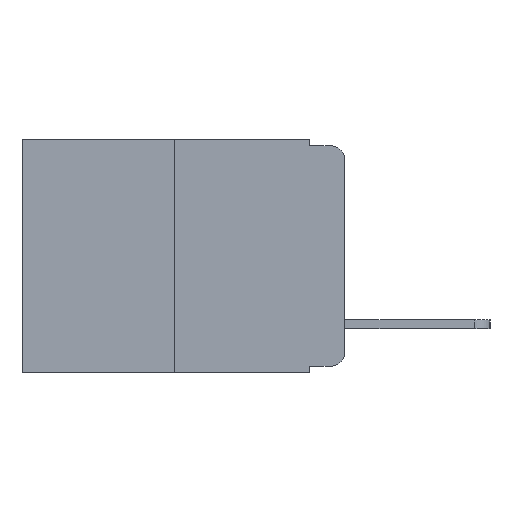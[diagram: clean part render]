
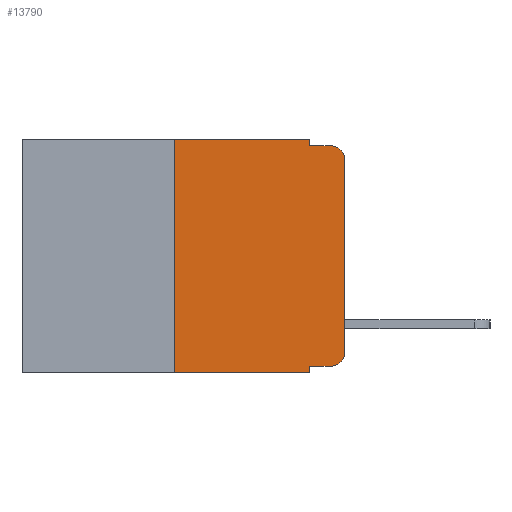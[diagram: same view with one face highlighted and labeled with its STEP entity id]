
A CAD part, left-side view. The second image highlights one B-rep face of the part: STEP entity #13790.
In plain terms, the highlighted planar face has unit normal (-1, 0, 0).
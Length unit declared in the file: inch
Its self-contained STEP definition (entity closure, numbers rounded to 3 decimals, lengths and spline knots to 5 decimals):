
#173 = CIRCLE ( 'NONE', #12057, 0.02 ) ;
#282 = CARTESIAN_POINT ( 'NONE',  ( 0., 0., 0. ) ) ;
#374 = CARTESIAN_POINT ( 'NONE',  ( 0., 0.473, 0. ) ) ;
#737 = ORIENTED_EDGE ( 'NONE', *, *, #6366, .T. ) ;
#846 = CARTESIAN_POINT ( 'NONE',  ( 0., 0.02, -0.313 ) ) ;
#1146 = DIRECTION ( 'NONE',  ( 0., -1., 0. ) ) ;
#1491 = ORIENTED_EDGE ( 'NONE', *, *, #15476, .F. ) ;
#1726 = VERTEX_POINT ( 'NONE', #10452 ) ;
#1946 = VERTEX_POINT ( 'NONE', #9944 ) ;
#1951 = CARTESIAN_POINT ( 'NONE',  ( 0., 0.051, 0. ) ) ;
#2490 = VECTOR ( 'NONE', #15350, 39.37008 ) ;
#2715 = DIRECTION ( 'NONE',  ( 0., 0., -1. ) ) ;
#2809 = CARTESIAN_POINT ( 'NONE',  ( 0., 0.473, -0.343 ) ) ;
#3084 = LINE ( 'NONE', #3645, #2490 ) ;
#3427 = DIRECTION ( 'NONE',  ( 0., -1., 0. ) ) ;
#3614 = CARTESIAN_POINT ( 'NONE',  ( 0., 0.02, -0.03 ) ) ;
#3626 = ORIENTED_EDGE ( 'NONE', *, *, #17528, .F. ) ;
#3645 = CARTESIAN_POINT ( 'NONE',  ( 0., 0.051, 0. ) ) ;
#3762 = DIRECTION ( 'NONE',  ( 0., 0., -1. ) ) ;
#4327 = LINE ( 'NONE', #16357, #4883 ) ;
#4883 = VECTOR ( 'NONE', #1146, 39.37008 ) ;
#4992 = PLANE ( 'NONE',  #20564 ) ;
#5311 = DIRECTION ( 'NONE',  ( 0., 0., -1. ) ) ;
#5549 = FACE_OUTER_BOUND ( 'NONE', #11961, .T. ) ;
#5662 = DIRECTION ( 'NONE',  ( 0., 0., 1. ) ) ;
#5912 = VERTEX_POINT ( 'NONE', #16687 ) ;
#6366 = EDGE_CURVE ( 'NONE', #12863, #11796, #8999, .T. ) ;
#6528 = VERTEX_POINT ( 'NONE', #21527 ) ;
#6591 = ORIENTED_EDGE ( 'NONE', *, *, #15136, .T. ) ;
#7450 = CARTESIAN_POINT ( 'NONE',  ( 0., 0.051, 0. ) ) ;
#7545 = VECTOR ( 'NONE', #5662, 39.37008 ) ;
#7729 = EDGE_CURVE ( 'NONE', #1946, #5912, #12686, .T. ) ;
#8394 = DIRECTION ( 'NONE',  ( 1., 0., 0. ) ) ;
#8600 = VERTEX_POINT ( 'NONE', #20666 ) ;
#8771 = EDGE_CURVE ( 'NONE', #8600, #11796, #19243, .T. ) ;
#8999 = LINE ( 'NONE', #2809, #16774 ) ;
#9052 = DIRECTION ( 'NONE',  ( 0., -1., 0. ) ) ;
#9218 = ORIENTED_EDGE ( 'NONE', *, *, #8771, .F. ) ;
#9636 = LINE ( 'NONE', #15212, #14551 ) ;
#9687 = ORIENTED_EDGE ( 'NONE', *, *, #19255, .F. ) ;
#9944 = CARTESIAN_POINT ( 'NONE',  ( 0., 0., -0.03 ) ) ;
#9951 = LINE ( 'NONE', #374, #13336 ) ;
#10452 = CARTESIAN_POINT ( 'NONE',  ( 0., 0., -0.313 ) ) ;
#10524 = ORIENTED_EDGE ( 'NONE', *, *, #12081, .T. ) ;
#10536 = VECTOR ( 'NONE', #3762, 39.37008 ) ;
#11796 = VERTEX_POINT ( 'NONE', #16002 ) ;
#11831 = AXIS2_PLACEMENT_3D ( 'NONE', #3614, #15311, #5311 ) ;
#11961 = EDGE_LOOP ( 'NONE', ( #19369, #20381, #9687, #1491, #3626, #14382, #737, #9218, #10524, #6591 ) ) ;
#12057 = AXIS2_PLACEMENT_3D ( 'NONE', #846, #12903, #2715 ) ;
#12066 = LINE ( 'NONE', #282, #7545 ) ;
#12081 = EDGE_CURVE ( 'NONE', #8600, #12145, #9636, .T. ) ;
#12145 = VERTEX_POINT ( 'NONE', #17055 ) ;
#12686 = CIRCLE ( 'NONE', #11831, 0.02 ) ;
#12863 = VERTEX_POINT ( 'NONE', #14185 ) ;
#12903 = DIRECTION ( 'NONE',  ( -1., 0., 0. ) ) ;
#13336 = VECTOR ( 'NONE', #9052, 39.37008 ) ;
#13764 = CARTESIAN_POINT ( 'NONE',  ( 0., 0.25, 0. ) ) ;
#13790 = ADVANCED_FACE ( 'NONE', ( #5549 ), #4992, .F. ) ;
#14185 = CARTESIAN_POINT ( 'NONE',  ( 0., 0.25, -0.343 ) ) ;
#14382 = ORIENTED_EDGE ( 'NONE', *, *, #14866, .F. ) ;
#14551 = VECTOR ( 'NONE', #3427, 39.37008 ) ;
#14866 = EDGE_CURVE ( 'NONE', #12863, #6528, #19519, .T. ) ;
#15136 = EDGE_CURVE ( 'NONE', #12145, #1726, #173, .T. ) ;
#15212 = CARTESIAN_POINT ( 'NONE',  ( 0., 0.051, -0.333 ) ) ;
#15264 = VERTEX_POINT ( 'NONE', #19640 ) ;
#15311 = DIRECTION ( 'NONE',  ( -1., 0., 0. ) ) ;
#15350 = DIRECTION ( 'NONE',  ( 0., 0., -1. ) ) ;
#15476 = EDGE_CURVE ( 'NONE', #17549, #15264, #3084, .T. ) ;
#16002 = CARTESIAN_POINT ( 'NONE',  ( 0., 0.051, -0.343 ) ) ;
#16357 = CARTESIAN_POINT ( 'NONE',  ( 0., 0.051, -0.01 ) ) ;
#16685 = EDGE_CURVE ( 'NONE', #1726, #1946, #12066, .T. ) ;
#16687 = CARTESIAN_POINT ( 'NONE',  ( 0., 0.02, -0.01 ) ) ;
#16774 = VECTOR ( 'NONE', #19509, 39.37008 ) ;
#17055 = CARTESIAN_POINT ( 'NONE',  ( 0., 0.02, -0.333 ) ) ;
#17528 = EDGE_CURVE ( 'NONE', #6528, #17549, #9951, .T. ) ;
#17549 = VERTEX_POINT ( 'NONE', #7450 ) ;
#18296 = CARTESIAN_POINT ( 'NONE',  ( 0., 0.473, 0. ) ) ;
#18659 = DIRECTION ( 'NONE',  ( 0., 0., 1. ) ) ;
#18987 = VECTOR ( 'NONE', #18659, 39.37008 ) ;
#19243 = LINE ( 'NONE', #1951, #10536 ) ;
#19255 = EDGE_CURVE ( 'NONE', #15264, #5912, #4327, .T. ) ;
#19369 = ORIENTED_EDGE ( 'NONE', *, *, #16685, .T. ) ;
#19509 = DIRECTION ( 'NONE',  ( 0., -1., 0. ) ) ;
#19519 = LINE ( 'NONE', #13764, #18987 ) ;
#19640 = CARTESIAN_POINT ( 'NONE',  ( 0., 0.051, -0.01 ) ) ;
#19927 = DIRECTION ( 'NONE',  ( 0., 0., -1. ) ) ;
#20381 = ORIENTED_EDGE ( 'NONE', *, *, #7729, .T. ) ;
#20564 = AXIS2_PLACEMENT_3D ( 'NONE', #18296, #8394, #19927 ) ;
#20666 = CARTESIAN_POINT ( 'NONE',  ( 0., 0.051, -0.333 ) ) ;
#21527 = CARTESIAN_POINT ( 'NONE',  ( 0., 0.25, 0. ) ) ;
